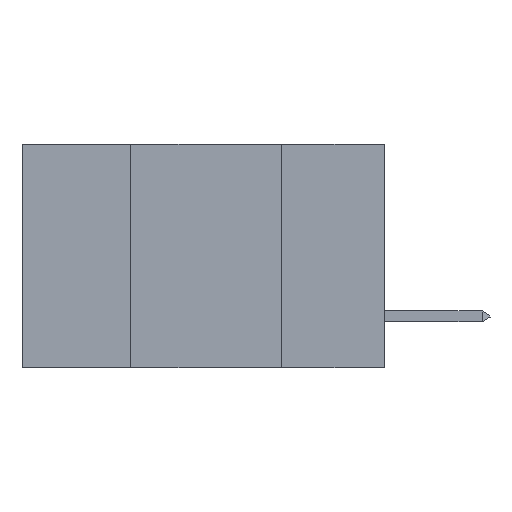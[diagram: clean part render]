
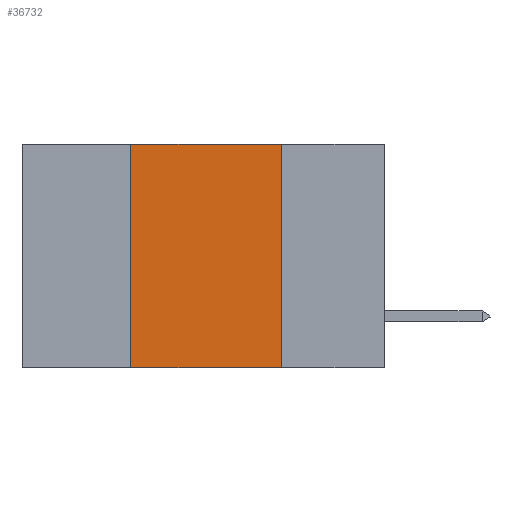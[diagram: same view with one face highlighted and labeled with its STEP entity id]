
A CAD part, left-side view. The second image highlights one B-rep face of the part: STEP entity #36732.
In plain terms, the highlighted planar face has unit normal (-1, 0, 0).
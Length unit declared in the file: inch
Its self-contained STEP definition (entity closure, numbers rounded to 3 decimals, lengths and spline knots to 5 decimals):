
#675 = DIRECTION ( 'NONE',  ( 0., 0., -1. ) ) ;
#1111 = ORIENTED_EDGE ( 'NONE', *, *, #47178, .F. ) ;
#1305 = PLANE ( 'NONE',  #13541 ) ;
#1349 = VERTEX_POINT ( 'NONE', #4187 ) ;
#1986 = ORIENTED_EDGE ( 'NONE', *, *, #34768, .F. ) ;
#3503 = DIRECTION ( 'NONE',  ( 0., -1., 0. ) ) ;
#3623 = VECTOR ( 'NONE', #22624, 39.37008 ) ;
#4187 = CARTESIAN_POINT ( 'NONE',  ( 0., 0.17, 0. ) ) ;
#4957 = DIRECTION ( 'NONE',  ( 1., 0., 0. ) ) ;
#6660 = FACE_OUTER_BOUND ( 'NONE', #24453, .T. ) ;
#6874 = LINE ( 'NONE', #33693, #31525 ) ;
#9530 = EDGE_CURVE ( 'NONE', #24089, #39434, #33421, .T. ) ;
#9936 = LINE ( 'NONE', #15038, #3623 ) ;
#11699 = CARTESIAN_POINT ( 'NONE',  ( 0., 0.42, -0.37 ) ) ;
#13541 = AXIS2_PLACEMENT_3D ( 'NONE', #23075, #4957, #675 ) ;
#14992 = CARTESIAN_POINT ( 'NONE',  ( 0., 0.42, 0. ) ) ;
#15038 = CARTESIAN_POINT ( 'NONE',  ( 0., 0.6, 0. ) ) ;
#18033 = ORIENTED_EDGE ( 'NONE', *, *, #9530, .T. ) ;
#18061 = DIRECTION ( 'NONE',  ( 0., 0., 1. ) ) ;
#20951 = CARTESIAN_POINT ( 'NONE',  ( 0., 0.17, -0.37 ) ) ;
#22062 = CARTESIAN_POINT ( 'NONE',  ( 0., 0.6, -0.37 ) ) ;
#22624 = DIRECTION ( 'NONE',  ( 0., -1., 0. ) ) ;
#22809 = DIRECTION ( 'NONE',  ( 0., 0., -1. ) ) ;
#23075 = CARTESIAN_POINT ( 'NONE',  ( 0., 0.6, 0. ) ) ;
#24089 = VERTEX_POINT ( 'NONE', #11699 ) ;
#24453 = EDGE_LOOP ( 'NONE', ( #1986, #27352, #1111, #18033 ) ) ;
#24846 = VECTOR ( 'NONE', #3503, 39.37008 ) ;
#26176 = LINE ( 'NONE', #14992, #44361 ) ;
#27352 = ORIENTED_EDGE ( 'NONE', *, *, #28950, .F. ) ;
#28950 = EDGE_CURVE ( 'NONE', #37886, #1349, #9936, .T. ) ;
#31525 = VECTOR ( 'NONE', #22809, 39.37008 ) ;
#32549 = CARTESIAN_POINT ( 'NONE',  ( 0., 0.42, 0. ) ) ;
#33421 = LINE ( 'NONE', #22062, #24846 ) ;
#33693 = CARTESIAN_POINT ( 'NONE',  ( 0., 0.17, 0. ) ) ;
#34768 = EDGE_CURVE ( 'NONE', #1349, #39434, #6874, .T. ) ;
#36732 = ADVANCED_FACE ( 'NONE', ( #6660 ), #1305, .F. ) ;
#37886 = VERTEX_POINT ( 'NONE', #32549 ) ;
#39434 = VERTEX_POINT ( 'NONE', #20951 ) ;
#44361 = VECTOR ( 'NONE', #18061, 39.37008 ) ;
#47178 = EDGE_CURVE ( 'NONE', #24089, #37886, #26176, .T. ) ;
